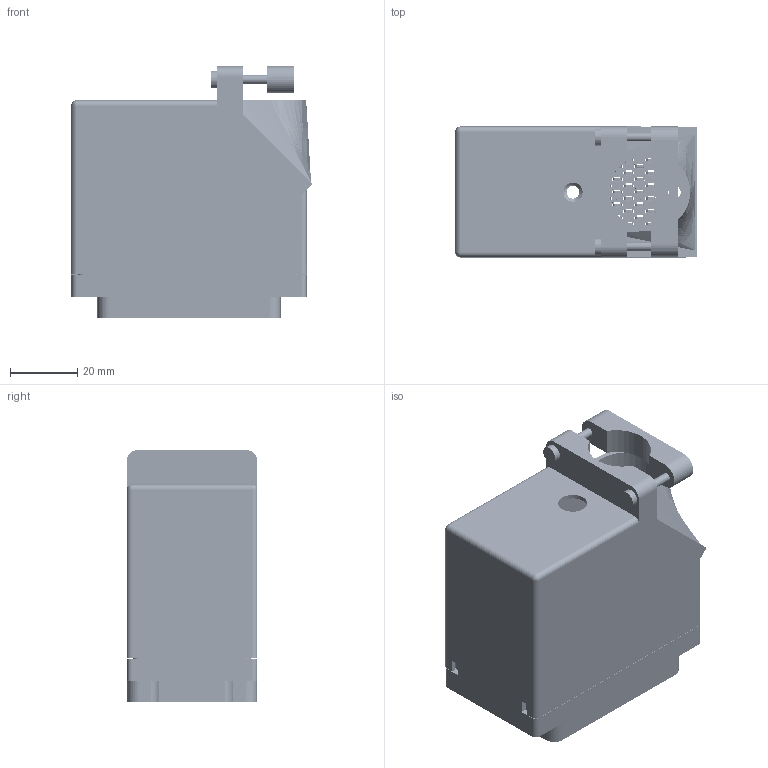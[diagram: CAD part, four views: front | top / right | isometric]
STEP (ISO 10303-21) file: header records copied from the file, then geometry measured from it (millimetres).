
FILE_DESCRIPTION (( 'STEP AP203' ), '1' );
FILE_NAME ('516-120-500-116.STEP', '2020-03-11T02:05:32', ( '' ), ( '' ), 'SwSTEP 2.0', 'SolidWorks 2016', '' );
FILE_SCHEMA (( 'CONFIG_CONTROL_DESIGN' ));
Length unit declared in the file: inch
Products named in the file (5): 516-292-001_500 Contact; 516-252-095-100; 516-120-500-116; 516 Plug Insulator_120; 516-230-001_Plastic - 120 Top Entry
Assembly tree (123 placements, depth 2):
  516-120-500-116
    516 Plug Insulator_120
    516-292-001_500 Contact  x120
    516-230-001_Plastic - 120 Top Entry
    516-252-095-100
Bounding box: 71.77 x 38.86 x 74.75 mm (x, y, z)
Volume: 46807 mm3; surface area: 76679.7 mm2
Topology: 123 solids, 123 shells, 11620 faces, 33809 edges, 22453 vertices
Faces by surface type: plane 7007, cylinder 3870, bspline 729, cone 12, sphere 2
Entity records: 93001 total; most frequent: CARTESIAN_POINT 17798, ORIENTED_EDGE 15254, DIRECTION 14699, EDGE_CURVE 7627, VECTOR 5757, LINE 5757, VERTEX_POINT 5079, AXIS2_PLACEMENT_3D 4471
